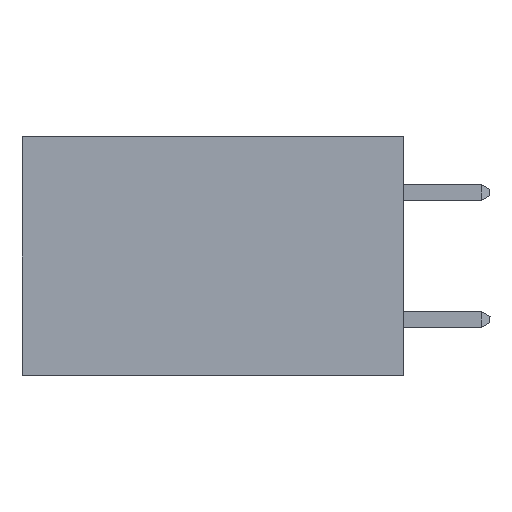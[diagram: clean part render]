
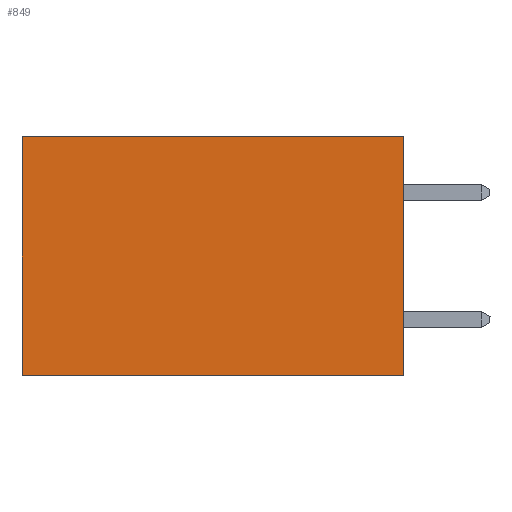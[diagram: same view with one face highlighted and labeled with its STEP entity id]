
A CAD part, left-side view. The second image highlights one B-rep face of the part: STEP entity #849.
In plain terms, the highlighted planar face has unit normal (-1, 0, 0).
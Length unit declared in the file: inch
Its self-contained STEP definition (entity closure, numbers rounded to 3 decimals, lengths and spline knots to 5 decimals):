
#176 = VECTOR ( 'NONE', #11606, 39.37008 ) ;
#444 = CARTESIAN_POINT ( 'NONE',  ( 0.2875, 0.6, -0.375 ) ) ;
#849 = ADVANCED_FACE ( 'NONE', ( #11080 ), #11215, .F. ) ;
#2153 = LINE ( 'NONE', #13260, #12939 ) ;
#2932 = EDGE_LOOP ( 'NONE', ( #11683, #9414, #12786, #12616 ) ) ;
#3043 = AXIS2_PLACEMENT_3D ( 'NONE', #7682, #12418, #11267 ) ;
#4462 = EDGE_CURVE ( 'NONE', #14384, #13621, #2153, .T. ) ;
#4554 = CARTESIAN_POINT ( 'NONE',  ( 0.2875, 0., 0. ) ) ;
#4712 = EDGE_CURVE ( 'NONE', #5511, #13621, #7540, .T. ) ;
#4781 = CARTESIAN_POINT ( 'NONE',  ( 0.2875, 0., 0. ) ) ;
#5511 = VERTEX_POINT ( 'NONE', #13203 ) ;
#5575 = LINE ( 'NONE', #12541, #7276 ) ;
#6587 = VECTOR ( 'NONE', #13775, 39.37008 ) ;
#6802 = EDGE_CURVE ( 'NONE', #13544, #14384, #8933, .T. ) ;
#7276 = VECTOR ( 'NONE', #14922, 39.37008 ) ;
#7540 = LINE ( 'NONE', #13928, #6587 ) ;
#7682 = CARTESIAN_POINT ( 'NONE',  ( 0.2875, 0., -0.375 ) ) ;
#8522 = DIRECTION ( 'NONE',  ( 0., 0., -1. ) ) ;
#8933 = LINE ( 'NONE', #4554, #176 ) ;
#9308 = CARTESIAN_POINT ( 'NONE',  ( 0.2875, 0.6, 0. ) ) ;
#9414 = ORIENTED_EDGE ( 'NONE', *, *, #4712, .F. ) ;
#10107 = EDGE_CURVE ( 'NONE', #13544, #5511, #5575, .T. ) ;
#11080 = FACE_OUTER_BOUND ( 'NONE', #2932, .T. ) ;
#11215 = PLANE ( 'NONE',  #3043 ) ;
#11267 = DIRECTION ( 'NONE',  ( 0., 0., -1. ) ) ;
#11606 = DIRECTION ( 'NONE',  ( 0., 1., 0. ) ) ;
#11683 = ORIENTED_EDGE ( 'NONE', *, *, #4462, .T. ) ;
#12418 = DIRECTION ( 'NONE',  ( 1., 0., 0. ) ) ;
#12541 = CARTESIAN_POINT ( 'NONE',  ( 0.2875, 0., -0.375 ) ) ;
#12616 = ORIENTED_EDGE ( 'NONE', *, *, #6802, .T. ) ;
#12786 = ORIENTED_EDGE ( 'NONE', *, *, #10107, .F. ) ;
#12939 = VECTOR ( 'NONE', #8522, 39.37008 ) ;
#13203 = CARTESIAN_POINT ( 'NONE',  ( 0.2875, 0., -0.375 ) ) ;
#13260 = CARTESIAN_POINT ( 'NONE',  ( 0.2875, 0.6, -0.375 ) ) ;
#13544 = VERTEX_POINT ( 'NONE', #4781 ) ;
#13621 = VERTEX_POINT ( 'NONE', #444 ) ;
#13775 = DIRECTION ( 'NONE',  ( 0., 1., 0. ) ) ;
#13928 = CARTESIAN_POINT ( 'NONE',  ( 0.2875, 0., -0.375 ) ) ;
#14384 = VERTEX_POINT ( 'NONE', #9308 ) ;
#14922 = DIRECTION ( 'NONE',  ( 0., 0., -1. ) ) ;
